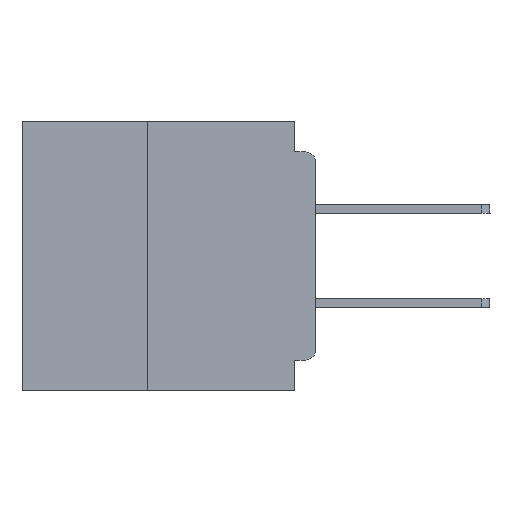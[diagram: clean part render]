
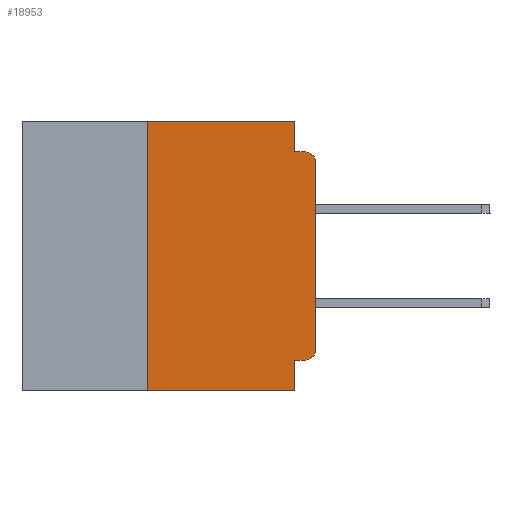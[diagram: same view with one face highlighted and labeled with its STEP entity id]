
A CAD part, left-side view. The second image highlights one B-rep face of the part: STEP entity #18953.
In plain terms, the highlighted planar face has unit normal (-1, 0, 0).
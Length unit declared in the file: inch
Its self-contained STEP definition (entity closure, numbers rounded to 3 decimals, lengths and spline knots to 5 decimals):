
#983 = LINE ( 'NONE', #53030, #53153 ) ;
#1870 = CARTESIAN_POINT ( 'NONE',  ( 0., 0., -0.045 ) ) ;
#3398 = CARTESIAN_POINT ( 'NONE',  ( 0., 0.437, 0. ) ) ;
#3682 = LINE ( 'NONE', #64584, #15675 ) ;
#4283 = DIRECTION ( 'NONE',  ( 0., 0., -1. ) ) ;
#4334 = VECTOR ( 'NONE', #59622, 39.37008 ) ;
#5917 = AXIS2_PLACEMENT_3D ( 'NONE', #9881, #45248, #14999 ) ;
#7022 = DIRECTION ( 'NONE',  ( 0., -1., 0. ) ) ;
#8047 = CARTESIAN_POINT ( 'NONE',  ( 0., 0.031, -0.4 ) ) ;
#8986 = VERTEX_POINT ( 'NONE', #33240 ) ;
#9639 = CARTESIAN_POINT ( 'NONE',  ( 0., 0.031, -0.355 ) ) ;
#9881 = CARTESIAN_POINT ( 'NONE',  ( 0., 0.015, -0.34 ) ) ;
#10295 = CIRCLE ( 'NONE', #5917, 0.015 ) ;
#10531 = EDGE_CURVE ( 'NONE', #43946, #8986, #63240, .T. ) ;
#12330 = VERTEX_POINT ( 'NONE', #37942 ) ;
#13043 = CARTESIAN_POINT ( 'NONE',  ( 0., 0., -0.34 ) ) ;
#13568 = VECTOR ( 'NONE', #63606, 39.37008 ) ;
#14393 = ORIENTED_EDGE ( 'NONE', *, *, #64560, .F. ) ;
#14456 = VERTEX_POINT ( 'NONE', #19529 ) ;
#14785 = ORIENTED_EDGE ( 'NONE', *, *, #10531, .T. ) ;
#14999 = DIRECTION ( 'NONE',  ( 0., 0., -1. ) ) ;
#15353 = EDGE_CURVE ( 'NONE', #47731, #48587, #56426, .T. ) ;
#15675 = VECTOR ( 'NONE', #4283, 39.37008 ) ;
#16307 = ORIENTED_EDGE ( 'NONE', *, *, #20933, .T. ) ;
#16312 = VECTOR ( 'NONE', #38341, 39.37008 ) ;
#17043 = CARTESIAN_POINT ( 'NONE',  ( 0., 0., -0.355 ) ) ;
#17084 = CARTESIAN_POINT ( 'NONE',  ( 0., 0.25, -0.4 ) ) ;
#17418 = FACE_OUTER_BOUND ( 'NONE', #49606, .T. ) ;
#17891 = EDGE_CURVE ( 'NONE', #61661, #48587, #28607, .T. ) ;
#18140 = CARTESIAN_POINT ( 'NONE',  ( 0., 0.015, -0.06 ) ) ;
#18408 = DIRECTION ( 'NONE',  ( 0., 0., 1. ) ) ;
#18953 = ADVANCED_FACE ( 'NONE', ( #17418 ), #48939, .F. ) ;
#19529 = CARTESIAN_POINT ( 'NONE',  ( 0., 0.031, 0. ) ) ;
#20777 = CARTESIAN_POINT ( 'NONE',  ( 0., 0.015, -0.355 ) ) ;
#20933 = EDGE_CURVE ( 'NONE', #21708, #61813, #10295, .T. ) ;
#21708 = VERTEX_POINT ( 'NONE', #20777 ) ;
#23180 = DIRECTION ( 'NONE',  ( 0., 0., -1. ) ) ;
#23817 = CARTESIAN_POINT ( 'NONE',  ( 0., 0., -0.06 ) ) ;
#23858 = DIRECTION ( 'NONE',  ( 0., 0., -1. ) ) ;
#24021 = ORIENTED_EDGE ( 'NONE', *, *, #62567, .F. ) ;
#25109 = LINE ( 'NONE', #17043, #65055 ) ;
#27083 = ORIENTED_EDGE ( 'NONE', *, *, #30984, .F. ) ;
#28547 = CARTESIAN_POINT ( 'NONE',  ( 0., 0., 0. ) ) ;
#28607 = LINE ( 'NONE', #58641, #13568 ) ;
#29024 = ORIENTED_EDGE ( 'NONE', *, *, #15353, .F. ) ;
#30984 = EDGE_CURVE ( 'NONE', #21708, #47731, #25109, .T. ) ;
#32619 = ORIENTED_EDGE ( 'NONE', *, *, #50528, .T. ) ;
#33240 = CARTESIAN_POINT ( 'NONE',  ( 0., 0.015, -0.045 ) ) ;
#33295 = VECTOR ( 'NONE', #18408, 39.37008 ) ;
#34655 = AXIS2_PLACEMENT_3D ( 'NONE', #18140, #53297, #23180 ) ;
#37458 = ORIENTED_EDGE ( 'NONE', *, *, #45970, .F. ) ;
#37942 = CARTESIAN_POINT ( 'NONE',  ( 0., 0.25, 0. ) ) ;
#38341 = DIRECTION ( 'NONE',  ( 0., 0., -1. ) ) ;
#41273 = ORIENTED_EDGE ( 'NONE', *, *, #62810, .F. ) ;
#41878 = AXIS2_PLACEMENT_3D ( 'NONE', #3398, #53980, #23858 ) ;
#41966 = DIRECTION ( 'NONE',  ( 0., 1., 0. ) ) ;
#43946 = VERTEX_POINT ( 'NONE', #23817 ) ;
#44739 = LINE ( 'NONE', #54626, #4334 ) ;
#45155 = LINE ( 'NONE', #28547, #33295 ) ;
#45176 = ORIENTED_EDGE ( 'NONE', *, *, #17891, .T. ) ;
#45248 = DIRECTION ( 'NONE',  ( -1., 0., 0. ) ) ;
#45970 = EDGE_CURVE ( 'NONE', #61661, #12330, #983, .T. ) ;
#46496 = LINE ( 'NONE', #1870, #58164 ) ;
#47731 = VERTEX_POINT ( 'NONE', #9639 ) ;
#48190 = DIRECTION ( 'NONE',  ( 0., 0., 1. ) ) ;
#48587 = VERTEX_POINT ( 'NONE', #61673 ) ;
#48939 = PLANE ( 'NONE',  #41878 ) ;
#49606 = EDGE_LOOP ( 'NONE', ( #32619, #14785, #24021, #41273, #14393, #37458, #45176, #29024, #27083, #16307 ) ) ;
#50510 = CARTESIAN_POINT ( 'NONE',  ( 0., 0.031, -0.045 ) ) ;
#50528 = EDGE_CURVE ( 'NONE', #61813, #43946, #45155, .T. ) ;
#53030 = CARTESIAN_POINT ( 'NONE',  ( 0., 0.25, -0.4 ) ) ;
#53153 = VECTOR ( 'NONE', #48190, 39.37008 ) ;
#53297 = DIRECTION ( 'NONE',  ( -1., 0., 0. ) ) ;
#53980 = DIRECTION ( 'NONE',  ( 1., 0., 0. ) ) ;
#54626 = CARTESIAN_POINT ( 'NONE',  ( 0., 0.437, 0. ) ) ;
#56017 = VERTEX_POINT ( 'NONE', #50510 ) ;
#56426 = LINE ( 'NONE', #8047, #16312 ) ;
#58164 = VECTOR ( 'NONE', #7022, 39.37008 ) ;
#58641 = CARTESIAN_POINT ( 'NONE',  ( 0., 0.437, -0.4 ) ) ;
#59622 = DIRECTION ( 'NONE',  ( 0., -1., 0. ) ) ;
#61661 = VERTEX_POINT ( 'NONE', #17084 ) ;
#61673 = CARTESIAN_POINT ( 'NONE',  ( 0., 0.031, -0.4 ) ) ;
#61813 = VERTEX_POINT ( 'NONE', #13043 ) ;
#62567 = EDGE_CURVE ( 'NONE', #56017, #8986, #46496, .T. ) ;
#62810 = EDGE_CURVE ( 'NONE', #14456, #56017, #3682, .T. ) ;
#63240 = CIRCLE ( 'NONE', #34655, 0.015 ) ;
#63606 = DIRECTION ( 'NONE',  ( 0., -1., 0. ) ) ;
#64560 = EDGE_CURVE ( 'NONE', #12330, #14456, #44739, .T. ) ;
#64584 = CARTESIAN_POINT ( 'NONE',  ( 0., 0.031, 0. ) ) ;
#65055 = VECTOR ( 'NONE', #41966, 39.37008 ) ;
